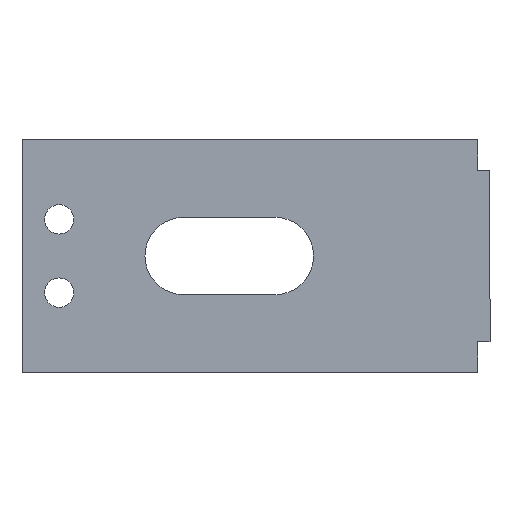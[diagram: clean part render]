
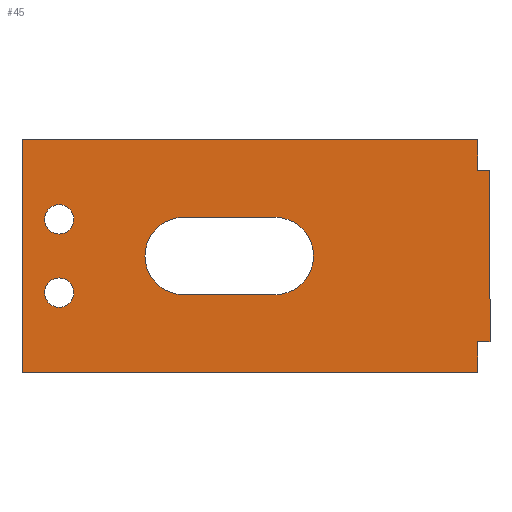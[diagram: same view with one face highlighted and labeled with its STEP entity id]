
A CAD part, front view. The second image highlights one B-rep face of the part: STEP entity #45.
In plain terms, the highlighted planar face has unit normal (0, -1, 0).
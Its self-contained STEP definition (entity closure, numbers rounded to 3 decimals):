
#7 = DIRECTION ( 'NONE',  ( 0., 0., 1. ) ) ;
#10 = CIRCLE ( 'NONE', #849, 3.97 ) ;
#12 = CARTESIAN_POINT ( 'NONE',  ( 3.81, -3.175, -8.188 ) ) ;
#27 = ORIENTED_EDGE ( 'NONE', *, *, #408, .T. ) ;
#31 = CARTESIAN_POINT ( 'NONE',  ( 0., -3.175, -15.908 ) ) ;
#38 = ORIENTED_EDGE ( 'NONE', *, *, #505, .T. ) ;
#45 = ADVANCED_FACE ( 'NONE', ( #149, #930, #152, #905 ), #943, .F. ) ;
#46 = ORIENTED_EDGE ( 'NONE', *, *, #683, .T. ) ;
#53 = CIRCLE ( 'NONE', #559, 1.5 ) ;
#57 = DIRECTION ( 'NONE',  ( 0., 0., 1. ) ) ;
#58 = AXIS2_PLACEMENT_3D ( 'NONE', #881, #452, #7 ) ;
#70 = VERTEX_POINT ( 'NONE', #133 ) ;
#77 = CIRCLE ( 'NONE', #898, 1.5 ) ;
#81 = DIRECTION ( 'NONE',  ( 1., 0., 0. ) ) ;
#84 = DIRECTION ( 'NONE',  ( 0., 0., 1. ) ) ;
#87 = DIRECTION ( 'NONE',  ( 0., 1., 0. ) ) ;
#91 = LINE ( 'NONE', #202, #662 ) ;
#92 = CARTESIAN_POINT ( 'NONE',  ( 16.568, -3.175, -15.908 ) ) ;
#132 = CARTESIAN_POINT ( 'NONE',  ( 16.568, -3.175, -11.938 ) ) ;
#133 = CARTESIAN_POINT ( 'NONE',  ( 46.685, -3.175, -23.876 ) ) ;
#137 = LINE ( 'NONE', #237, #889 ) ;
#149 = FACE_OUTER_BOUND ( 'NONE', #784, .T. ) ;
#152 = FACE_BOUND ( 'NONE', #287, .T. ) ;
#168 = VECTOR ( 'NONE', #323, 1000. ) ;
#171 = DIRECTION ( 'NONE',  ( 1., 0., 0. ) ) ;
#177 = DIRECTION ( 'NONE',  ( 0., 0., -1. ) ) ;
#194 = EDGE_CURVE ( 'NONE', #598, #289, #10, .T. ) ;
#197 = VECTOR ( 'NONE', #433, 1000. ) ;
#199 = ORIENTED_EDGE ( 'NONE', *, *, #872, .F. ) ;
#202 = CARTESIAN_POINT ( 'NONE',  ( 0., -3.175, -20.701 ) ) ;
#210 = DIRECTION ( 'NONE',  ( 0., 0., 1. ) ) ;
#215 = LINE ( 'NONE', #393, #590 ) ;
#226 = EDGE_CURVE ( 'NONE', #730, #754, #379, .T. ) ;
#229 = CARTESIAN_POINT ( 'NONE',  ( 3.81, -3.175, -15.688 ) ) ;
#237 = CARTESIAN_POINT ( 'NONE',  ( 0., -3.175, -7.968 ) ) ;
#249 = ORIENTED_EDGE ( 'NONE', *, *, #396, .F. ) ;
#264 = ORIENTED_EDGE ( 'NONE', *, *, #525, .F. ) ;
#275 = DIRECTION ( 'NONE',  ( 1., 0., 0. ) ) ;
#281 = CARTESIAN_POINT ( 'NONE',  ( 0., -3.175, -3.175 ) ) ;
#287 = EDGE_LOOP ( 'NONE', ( #606, #497 ) ) ;
#288 = CARTESIAN_POINT ( 'NONE',  ( 25.903, -3.175, -7.968 ) ) ;
#289 = VERTEX_POINT ( 'NONE', #440 ) ;
#304 = DIRECTION ( 'NONE',  ( 0., 0., 1. ) ) ;
#315 = CARTESIAN_POINT ( 'NONE',  ( 46.685, -3.175, 0. ) ) ;
#320 = VECTOR ( 'NONE', #700, 1000. ) ;
#323 = DIRECTION ( 'NONE',  ( 1., 0., 0. ) ) ;
#330 = CARTESIAN_POINT ( 'NONE',  ( 25.903, -3.175, -15.908 ) ) ;
#338 = EDGE_CURVE ( 'NONE', #809, #728, #91, .T. ) ;
#357 = VERTEX_POINT ( 'NONE', #665 ) ;
#371 = CARTESIAN_POINT ( 'NONE',  ( 3.81, -3.175, -9.688 ) ) ;
#375 = CARTESIAN_POINT ( 'NONE',  ( 0., -3.175, 0. ) ) ;
#379 = LINE ( 'NONE', #721, #936 ) ;
#383 = AXIS2_PLACEMENT_3D ( 'NONE', #795, #504, #653 ) ;
#388 = EDGE_CURVE ( 'NONE', #434, #479, #415, .T. ) ;
#390 = VECTOR ( 'NONE', #586, 1000. ) ;
#391 = VERTEX_POINT ( 'NONE', #797 ) ;
#393 = CARTESIAN_POINT ( 'NONE',  ( 0., -3.175, 0. ) ) ;
#395 = CARTESIAN_POINT ( 'NONE',  ( 46.685, -3.175, -20.701 ) ) ;
#396 = EDGE_CURVE ( 'NONE', #730, #707, #593, .T. ) ;
#402 = ORIENTED_EDGE ( 'NONE', *, *, #194, .T. ) ;
#406 = ORIENTED_EDGE ( 'NONE', *, *, #226, .T. ) ;
#408 = EDGE_CURVE ( 'NONE', #70, #809, #805, .T. ) ;
#415 = CIRCLE ( 'NONE', #922, 1.5 ) ;
#418 = VERTEX_POINT ( 'NONE', #288 ) ;
#430 = DIRECTION ( 'NONE',  ( 0., 1., 0. ) ) ;
#433 = DIRECTION ( 'NONE',  ( 0., 0., 1. ) ) ;
#434 = VERTEX_POINT ( 'NONE', #514 ) ;
#439 = VERTEX_POINT ( 'NONE', #517 ) ;
#440 = CARTESIAN_POINT ( 'NONE',  ( 16.568, -3.175, -7.968 ) ) ;
#452 = DIRECTION ( 'NONE',  ( 0., 1., 0. ) ) ;
#459 = CARTESIAN_POINT ( 'NONE',  ( 46.685, -3.175, -3.175 ) ) ;
#467 = CARTESIAN_POINT ( 'NONE',  ( 0., -3.175, -23.876 ) ) ;
#476 = CIRCLE ( 'NONE', #58, 3.97 ) ;
#479 = VERTEX_POINT ( 'NONE', #371 ) ;
#489 = EDGE_LOOP ( 'NONE', ( #38, #705 ) ) ;
#497 = ORIENTED_EDGE ( 'NONE', *, *, #546, .T. ) ;
#504 = DIRECTION ( 'NONE',  ( 0., 1., 0. ) ) ;
#505 = EDGE_CURVE ( 'NONE', #439, #357, #693, .T. ) ;
#510 = EDGE_CURVE ( 'NONE', #418, #914, #476, .T. ) ;
#514 = CARTESIAN_POINT ( 'NONE',  ( 3.81, -3.175, -6.688 ) ) ;
#517 = CARTESIAN_POINT ( 'NONE',  ( 3.81, -3.175, -14.188 ) ) ;
#518 = LINE ( 'NONE', #692, #320 ) ;
#525 = EDGE_CURVE ( 'NONE', #647, #754, #834, .T. ) ;
#529 = CARTESIAN_POINT ( 'NONE',  ( 0., -3.175, 0. ) ) ;
#530 = DIRECTION ( 'NONE',  ( 0., 1., 0. ) ) ;
#535 = CARTESIAN_POINT ( 'NONE',  ( 3.81, -3.175, -15.688 ) ) ;
#546 = EDGE_CURVE ( 'NONE', #479, #434, #77, .T. ) ;
#559 = AXIS2_PLACEMENT_3D ( 'NONE', #535, #87, #610 ) ;
#566 = EDGE_CURVE ( 'NONE', #357, #439, #53, .T. ) ;
#569 = LINE ( 'NONE', #31, #168 ) ;
#586 = DIRECTION ( 'NONE',  ( 1., 0., 0. ) ) ;
#590 = VECTOR ( 'NONE', #177, 1000. ) ;
#593 = LINE ( 'NONE', #281, #390 ) ;
#598 = VERTEX_POINT ( 'NONE', #92 ) ;
#606 = ORIENTED_EDGE ( 'NONE', *, *, #388, .T. ) ;
#610 = DIRECTION ( 'NONE',  ( 0., 0., 1. ) ) ;
#618 = EDGE_LOOP ( 'NONE', ( #867, #810, #402, #46 ) ) ;
#635 = EDGE_CURVE ( 'NONE', #391, #70, #935, .T. ) ;
#645 = VECTOR ( 'NONE', #81, 1000. ) ;
#647 = VERTEX_POINT ( 'NONE', #529 ) ;
#652 = DIRECTION ( 'NONE',  ( 0., 1., 0. ) ) ;
#653 = DIRECTION ( 'NONE',  ( 0., 0., 1. ) ) ;
#662 = VECTOR ( 'NONE', #275, 1000. ) ;
#665 = CARTESIAN_POINT ( 'NONE',  ( 3.81, -3.175, -17.188 ) ) ;
#670 = ORIENTED_EDGE ( 'NONE', *, *, #635, .T. ) ;
#679 = CARTESIAN_POINT ( 'NONE',  ( 47.955, -3.175, -3.175 ) ) ;
#683 = EDGE_CURVE ( 'NONE', #289, #418, #137, .T. ) ;
#692 = CARTESIAN_POINT ( 'NONE',  ( 47.955, -3.175, 0. ) ) ;
#693 = CIRCLE ( 'NONE', #840, 1.5 ) ;
#700 = DIRECTION ( 'NONE',  ( 0., 0., -1. ) ) ;
#705 = ORIENTED_EDGE ( 'NONE', *, *, #566, .T. ) ;
#707 = VERTEX_POINT ( 'NONE', #679 ) ;
#721 = CARTESIAN_POINT ( 'NONE',  ( 46.685, -3.175, 0. ) ) ;
#728 = VERTEX_POINT ( 'NONE', #891 ) ;
#730 = VERTEX_POINT ( 'NONE', #459 ) ;
#744 = DIRECTION ( 'NONE',  ( 0., 1., 0. ) ) ;
#748 = VECTOR ( 'NONE', #171, 1000. ) ;
#754 = VERTEX_POINT ( 'NONE', #315 ) ;
#783 = EDGE_CURVE ( 'NONE', #647, #391, #215, .T. ) ;
#784 = EDGE_LOOP ( 'NONE', ( #919, #670, #27, #835, #199, #249, #406, #264 ) ) ;
#795 = CARTESIAN_POINT ( 'NONE',  ( 0., -3.175, 0. ) ) ;
#797 = CARTESIAN_POINT ( 'NONE',  ( 0., -3.175, -23.876 ) ) ;
#803 = EDGE_CURVE ( 'NONE', #598, #914, #569, .T. ) ;
#805 = LINE ( 'NONE', #944, #197 ) ;
#809 = VERTEX_POINT ( 'NONE', #395 ) ;
#810 = ORIENTED_EDGE ( 'NONE', *, *, #803, .F. ) ;
#817 = DIRECTION ( 'NONE',  ( 1., 0., 0. ) ) ;
#834 = LINE ( 'NONE', #375, #645 ) ;
#835 = ORIENTED_EDGE ( 'NONE', *, *, #338, .T. ) ;
#840 = AXIS2_PLACEMENT_3D ( 'NONE', #229, #744, #304 ) ;
#849 = AXIS2_PLACEMENT_3D ( 'NONE', #132, #652, #210 ) ;
#858 = CARTESIAN_POINT ( 'NONE',  ( 3.81, -3.175, -8.188 ) ) ;
#867 = ORIENTED_EDGE ( 'NONE', *, *, #510, .T. ) ;
#872 = EDGE_CURVE ( 'NONE', #707, #728, #518, .T. ) ;
#881 = CARTESIAN_POINT ( 'NONE',  ( 25.903, -3.175, -11.938 ) ) ;
#889 = VECTOR ( 'NONE', #817, 1000. ) ;
#891 = CARTESIAN_POINT ( 'NONE',  ( 47.955, -3.175, -20.701 ) ) ;
#898 = AXIS2_PLACEMENT_3D ( 'NONE', #12, #530, #84 ) ;
#905 = FACE_BOUND ( 'NONE', #489, .T. ) ;
#914 = VERTEX_POINT ( 'NONE', #330 ) ;
#919 = ORIENTED_EDGE ( 'NONE', *, *, #783, .T. ) ;
#922 = AXIS2_PLACEMENT_3D ( 'NONE', #858, #430, #940 ) ;
#930 = FACE_BOUND ( 'NONE', #618, .T. ) ;
#935 = LINE ( 'NONE', #467, #748 ) ;
#936 = VECTOR ( 'NONE', #57, 1000. ) ;
#940 = DIRECTION ( 'NONE',  ( 0., 0., 1. ) ) ;
#943 = PLANE ( 'NONE',  #383 ) ;
#944 = CARTESIAN_POINT ( 'NONE',  ( 46.685, -3.175, 0. ) ) ;
